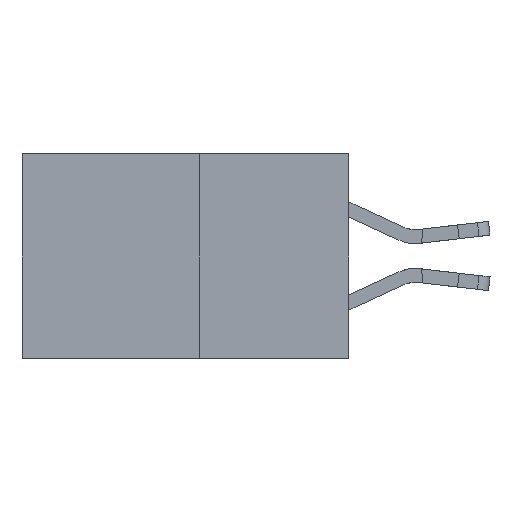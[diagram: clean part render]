
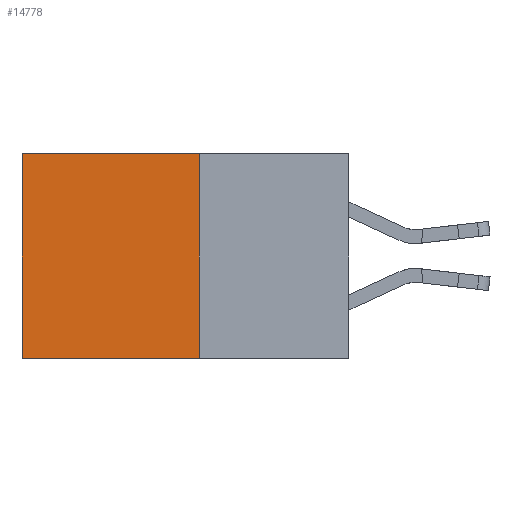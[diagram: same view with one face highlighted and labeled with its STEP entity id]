
A CAD part, left-side view. The second image highlights one B-rep face of the part: STEP entity #14778.
In plain terms, the highlighted planar face has unit normal (-1, 0, 0).
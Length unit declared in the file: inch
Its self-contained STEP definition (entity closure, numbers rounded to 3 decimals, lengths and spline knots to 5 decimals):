
#652 = CARTESIAN_POINT ( 'NONE',  ( 0.277, 0.27, -0.37 ) ) ;
#1740 = VECTOR ( 'NONE', #3691, 39.37008 ) ;
#1834 = DIRECTION ( 'NONE',  ( 0., 1., 0. ) ) ;
#1961 = ORIENTED_EDGE ( 'NONE', *, *, #9128, .T. ) ;
#1992 = PLANE ( 'NONE',  #5006 ) ;
#2354 = CARTESIAN_POINT ( 'NONE',  ( 0.277, 0.27, -0.37 ) ) ;
#2590 = EDGE_CURVE ( 'NONE', #16204, #4691, #16099, .T. ) ;
#3278 = VECTOR ( 'NONE', #13953, 39.37008 ) ;
#3330 = DIRECTION ( 'NONE',  ( 1., 0., 0. ) ) ;
#3661 = CARTESIAN_POINT ( 'NONE',  ( 0.277, 0.27, -0.37 ) ) ;
#3691 = DIRECTION ( 'NONE',  ( 0., 1., 0. ) ) ;
#3844 = VECTOR ( 'NONE', #1834, 39.37008 ) ;
#4097 = EDGE_CURVE ( 'NONE', #10875, #11752, #15051, .T. ) ;
#4691 = VERTEX_POINT ( 'NONE', #8160 ) ;
#5006 = AXIS2_PLACEMENT_3D ( 'NONE', #652, #3330, #12786 ) ;
#5142 = CARTESIAN_POINT ( 'NONE',  ( 0.277, 0.59, -0.37 ) ) ;
#5547 = LINE ( 'NONE', #12698, #12353 ) ;
#5919 = DIRECTION ( 'NONE',  ( 0., 0., -1. ) ) ;
#6404 = LINE ( 'NONE', #5142, #3278 ) ;
#7016 = ORIENTED_EDGE ( 'NONE', *, *, #4097, .T. ) ;
#7143 = EDGE_LOOP ( 'NONE', ( #1961, #13697, #7248, #7016 ) ) ;
#7248 = ORIENTED_EDGE ( 'NONE', *, *, #9170, .F. ) ;
#8160 = CARTESIAN_POINT ( 'NONE',  ( 0.277, 0.59, -0.37 ) ) ;
#9128 = EDGE_CURVE ( 'NONE', #11752, #4691, #6404, .T. ) ;
#9170 = EDGE_CURVE ( 'NONE', #10875, #16204, #5547, .T. ) ;
#10875 = VERTEX_POINT ( 'NONE', #16300 ) ;
#11432 = CARTESIAN_POINT ( 'NONE',  ( 0.277, 0.59, 0. ) ) ;
#11752 = VERTEX_POINT ( 'NONE', #11432 ) ;
#12353 = VECTOR ( 'NONE', #5919, 39.37008 ) ;
#12698 = CARTESIAN_POINT ( 'NONE',  ( 0.277, 0.27, -0.37 ) ) ;
#12786 = DIRECTION ( 'NONE',  ( 0., 0., -1. ) ) ;
#13697 = ORIENTED_EDGE ( 'NONE', *, *, #2590, .F. ) ;
#13953 = DIRECTION ( 'NONE',  ( 0., 0., -1. ) ) ;
#14778 = ADVANCED_FACE ( 'NONE', ( #16569 ), #1992, .F. ) ;
#15051 = LINE ( 'NONE', #16760, #3844 ) ;
#16099 = LINE ( 'NONE', #2354, #1740 ) ;
#16204 = VERTEX_POINT ( 'NONE', #3661 ) ;
#16300 = CARTESIAN_POINT ( 'NONE',  ( 0.277, 0.27, 0. ) ) ;
#16569 = FACE_OUTER_BOUND ( 'NONE', #7143, .T. ) ;
#16760 = CARTESIAN_POINT ( 'NONE',  ( 0.277, 0.27, 0. ) ) ;
